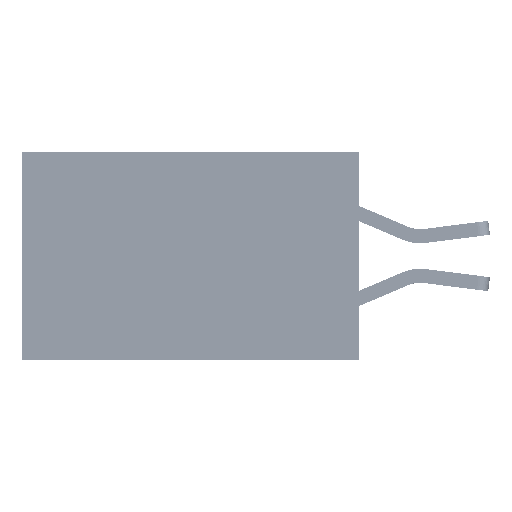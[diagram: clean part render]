
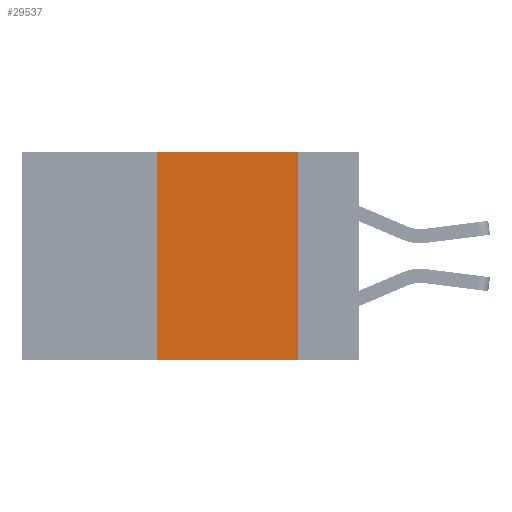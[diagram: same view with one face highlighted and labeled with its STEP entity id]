
A CAD part, left-side view. The second image highlights one B-rep face of the part: STEP entity #29537.
In plain terms, the highlighted planar face has unit normal (-1, 0, 0).
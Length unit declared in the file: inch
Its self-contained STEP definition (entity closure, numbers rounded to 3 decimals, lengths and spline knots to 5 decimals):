
#1427 = EDGE_CURVE ( 'NONE', #2463, #13051, #10526, .T. ) ;
#1611 = DIRECTION ( 'NONE',  ( 0., -1., 0. ) ) ;
#1738 = DIRECTION ( 'NONE',  ( 0., 0., -1. ) ) ;
#2463 = VERTEX_POINT ( 'NONE', #38409 ) ;
#2928 = DIRECTION ( 'NONE',  ( 0., -1., 0. ) ) ;
#4735 = LINE ( 'NONE', #20844, #38413 ) ;
#6745 = CARTESIAN_POINT ( 'NONE',  ( 0., 0.11, -0.37 ) ) ;
#7598 = CARTESIAN_POINT ( 'NONE',  ( 0., 0.36, 0. ) ) ;
#8477 = DIRECTION ( 'NONE',  ( 1., 0., 0. ) ) ;
#8955 = DIRECTION ( 'NONE',  ( 0., 0., 1. ) ) ;
#10526 = LINE ( 'NONE', #23816, #16069 ) ;
#11049 = DIRECTION ( 'NONE',  ( 0., 0., -1. ) ) ;
#13051 = VERTEX_POINT ( 'NONE', #6745 ) ;
#14868 = ORIENTED_EDGE ( 'NONE', *, *, #34663, .F. ) ;
#15178 = CARTESIAN_POINT ( 'NONE',  ( 0., 0.11, 0. ) ) ;
#15246 = ORIENTED_EDGE ( 'NONE', *, *, #36043, .F. ) ;
#15489 = VECTOR ( 'NONE', #8955, 39.37008 ) ;
#16069 = VECTOR ( 'NONE', #2928, 39.37008 ) ;
#16298 = AXIS2_PLACEMENT_3D ( 'NONE', #31348, #8477, #1738 ) ;
#18423 = ORIENTED_EDGE ( 'NONE', *, *, #1427, .T. ) ;
#18752 = CARTESIAN_POINT ( 'NONE',  ( 0., 0.36, 0. ) ) ;
#20844 = CARTESIAN_POINT ( 'NONE',  ( 0., 0.11, 0. ) ) ;
#22454 = LINE ( 'NONE', #18752, #15489 ) ;
#23257 = VECTOR ( 'NONE', #1611, 39.37008 ) ;
#23816 = CARTESIAN_POINT ( 'NONE',  ( 0., 0.6, -0.37 ) ) ;
#24208 = EDGE_LOOP ( 'NONE', ( #14868, #15246, #28430, #18423 ) ) ;
#24913 = VERTEX_POINT ( 'NONE', #15178 ) ;
#28006 = EDGE_CURVE ( 'NONE', #2463, #31650, #22454, .T. ) ;
#28430 = ORIENTED_EDGE ( 'NONE', *, *, #28006, .F. ) ;
#29537 = ADVANCED_FACE ( 'NONE', ( #31559 ), #41129, .F. ) ;
#31348 = CARTESIAN_POINT ( 'NONE',  ( 0., 0.6, 0. ) ) ;
#31559 = FACE_OUTER_BOUND ( 'NONE', #24208, .T. ) ;
#31650 = VERTEX_POINT ( 'NONE', #7598 ) ;
#34663 = EDGE_CURVE ( 'NONE', #24913, #13051, #4735, .T. ) ;
#36043 = EDGE_CURVE ( 'NONE', #31650, #24913, #40570, .T. ) ;
#38409 = CARTESIAN_POINT ( 'NONE',  ( 0., 0.36, -0.37 ) ) ;
#38413 = VECTOR ( 'NONE', #11049, 39.37008 ) ;
#40570 = LINE ( 'NONE', #40786, #23257 ) ;
#40786 = CARTESIAN_POINT ( 'NONE',  ( 0., 0.6, 0. ) ) ;
#41129 = PLANE ( 'NONE',  #16298 ) ;
